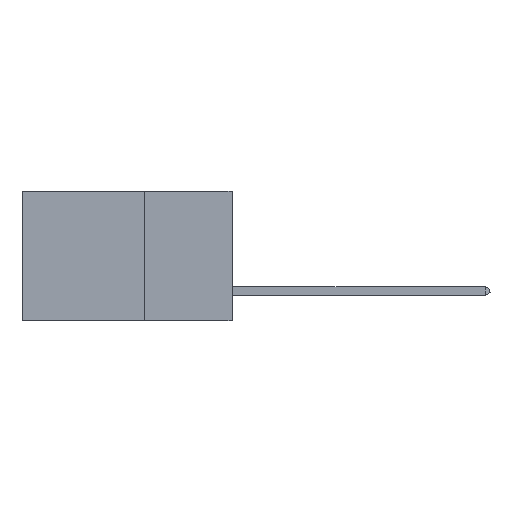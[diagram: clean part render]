
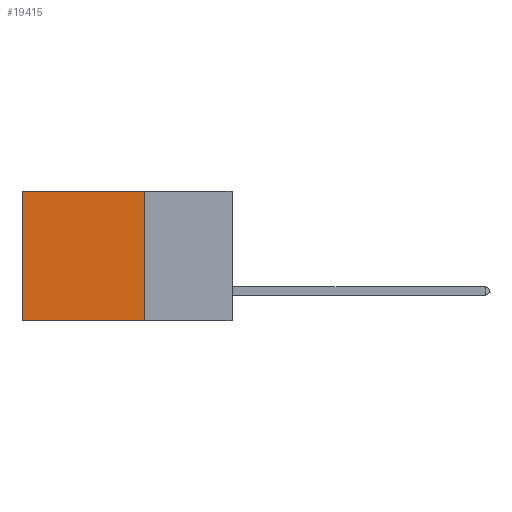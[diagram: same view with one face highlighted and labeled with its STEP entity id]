
A CAD part, left-side view. The second image highlights one B-rep face of the part: STEP entity #19415.
In plain terms, the highlighted planar face has unit normal (-1, 0, 0).
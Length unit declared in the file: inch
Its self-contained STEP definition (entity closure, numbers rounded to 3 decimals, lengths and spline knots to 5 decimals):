
#3930 = VERTEX_POINT ( 'NONE', #25528 ) ;
#4159 = EDGE_CURVE ( 'NONE', #4891, #30559, #11778, .T. ) ;
#4235 = DIRECTION ( 'NONE',  ( 0., 1., 0. ) ) ;
#4891 = VERTEX_POINT ( 'NONE', #26454 ) ;
#6063 = AXIS2_PLACEMENT_3D ( 'NONE', #29293, #19927, #13290 ) ;
#7860 = VECTOR ( 'NONE', #27779, 39.37008 ) ;
#8431 = CARTESIAN_POINT ( 'NONE',  ( 0.2875, 0.25, 0. ) ) ;
#9086 = CARTESIAN_POINT ( 'NONE',  ( 0.2875, 0.25, 0. ) ) ;
#10465 = ORIENTED_EDGE ( 'NONE', *, *, #4159, .F. ) ;
#11778 = LINE ( 'NONE', #9086, #7860 ) ;
#13211 = EDGE_LOOP ( 'NONE', ( #33242, #24757, #10465, #25152 ) ) ;
#13290 = DIRECTION ( 'NONE',  ( 0., 0., -1. ) ) ;
#13749 = VECTOR ( 'NONE', #33813, 39.37008 ) ;
#14671 = EDGE_CURVE ( 'NONE', #30559, #15029, #32102, .T. ) ;
#15029 = VERTEX_POINT ( 'NONE', #31450 ) ;
#16193 = FACE_OUTER_BOUND ( 'NONE', #13211, .T. ) ;
#18006 = CARTESIAN_POINT ( 'NONE',  ( 0.2875, 0.25, -0.37 ) ) ;
#18616 = CARTESIAN_POINT ( 'NONE',  ( 0.2875, 0.6, 0. ) ) ;
#19415 = ADVANCED_FACE ( 'NONE', ( #16193 ), #19727, .F. ) ;
#19618 = VECTOR ( 'NONE', #36499, 39.37008 ) ;
#19727 = PLANE ( 'NONE',  #6063 ) ;
#19927 = DIRECTION ( 'NONE',  ( 1., 0., 0. ) ) ;
#21330 = LINE ( 'NONE', #18616, #13749 ) ;
#24757 = ORIENTED_EDGE ( 'NONE', *, *, #14671, .F. ) ;
#25152 = ORIENTED_EDGE ( 'NONE', *, *, #33901, .T. ) ;
#25528 = CARTESIAN_POINT ( 'NONE',  ( 0.2875, 0.6, 0. ) ) ;
#26454 = CARTESIAN_POINT ( 'NONE',  ( 0.2875, 0.25, 0. ) ) ;
#27779 = DIRECTION ( 'NONE',  ( 0., 0., -1. ) ) ;
#28999 = CARTESIAN_POINT ( 'NONE',  ( 0.2875, 0.25, -0.37 ) ) ;
#29083 = VECTOR ( 'NONE', #4235, 39.37008 ) ;
#29293 = CARTESIAN_POINT ( 'NONE',  ( 0.2875, 0.25, 0. ) ) ;
#30475 = EDGE_CURVE ( 'NONE', #3930, #15029, #21330, .T. ) ;
#30559 = VERTEX_POINT ( 'NONE', #18006 ) ;
#31450 = CARTESIAN_POINT ( 'NONE',  ( 0.2875, 0.6, -0.37 ) ) ;
#32102 = LINE ( 'NONE', #28999, #29083 ) ;
#33242 = ORIENTED_EDGE ( 'NONE', *, *, #30475, .T. ) ;
#33813 = DIRECTION ( 'NONE',  ( 0., 0., -1. ) ) ;
#33901 = EDGE_CURVE ( 'NONE', #4891, #3930, #36898, .T. ) ;
#36499 = DIRECTION ( 'NONE',  ( 0., 1., 0. ) ) ;
#36898 = LINE ( 'NONE', #8431, #19618 ) ;
